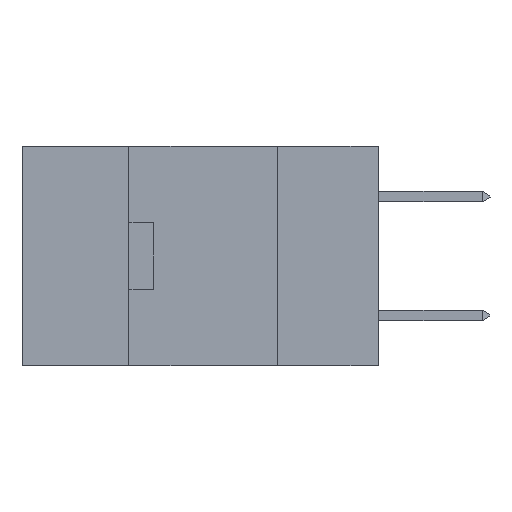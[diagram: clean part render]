
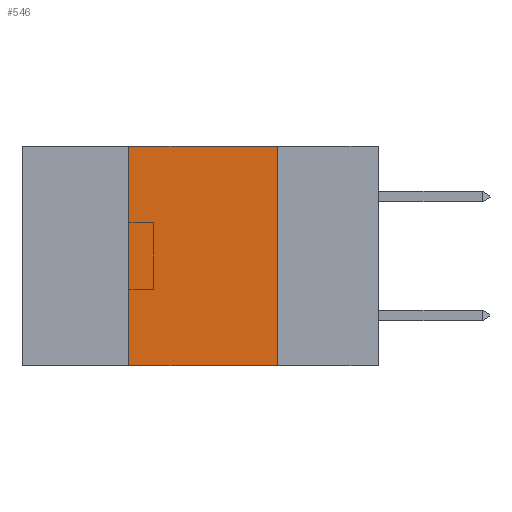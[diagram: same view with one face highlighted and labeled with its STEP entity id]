
A CAD part, left-side view. The second image highlights one B-rep face of the part: STEP entity #546.
In plain terms, the highlighted planar face has unit normal (-1, 0, 0).
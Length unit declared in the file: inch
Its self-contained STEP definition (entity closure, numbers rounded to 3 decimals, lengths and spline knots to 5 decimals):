
#224 = EDGE_CURVE ( 'NONE', #2833, #1646, #24307, .T. ) ;
#247 = VECTOR ( 'NONE', #17363, 39.37008 ) ;
#546 = ADVANCED_FACE ( 'NONE', ( #5704 ), #17321, .F. ) ;
#1470 = VERTEX_POINT ( 'NONE', #16471 ) ;
#1646 = VERTEX_POINT ( 'NONE', #10199 ) ;
#2113 = CARTESIAN_POINT ( 'NONE',  ( 0., 0.6, 0. ) ) ;
#2207 = DIRECTION ( 'NONE',  ( 0., -1., 0. ) ) ;
#2833 = VERTEX_POINT ( 'NONE', #9070 ) ;
#4577 = LINE ( 'NONE', #2113, #27231 ) ;
#5086 = AXIS2_PLACEMENT_3D ( 'NONE', #17224, #17189, #17125 ) ;
#5297 = ORIENTED_EDGE ( 'NONE', *, *, #15678, .F. ) ;
#5704 = FACE_OUTER_BOUND ( 'NONE', #21812, .T. ) ;
#6000 = ORIENTED_EDGE ( 'NONE', *, *, #16974, .F. ) ;
#7473 = DIRECTION ( 'NONE',  ( 0., 0., 1. ) ) ;
#9070 = CARTESIAN_POINT ( 'NONE',  ( 0., 0.42, -0.37 ) ) ;
#9795 = ORIENTED_EDGE ( 'NONE', *, *, #25012, .T. ) ;
#10057 = CARTESIAN_POINT ( 'NONE',  ( 0., 0.42, -0.37 ) ) ;
#10199 = CARTESIAN_POINT ( 'NONE',  ( 0., 0.42, 0. ) ) ;
#12077 = LINE ( 'NONE', #23946, #247 ) ;
#12909 = CARTESIAN_POINT ( 'NONE',  ( 0., 0.17, 0. ) ) ;
#15678 = EDGE_CURVE ( 'NONE', #1646, #18724, #4577, .T. ) ;
#16471 = CARTESIAN_POINT ( 'NONE',  ( 0., 0.17, -0.37 ) ) ;
#16974 = EDGE_CURVE ( 'NONE', #18724, #1470, #12077, .T. ) ;
#17125 = DIRECTION ( 'NONE',  ( 0., 0., -1. ) ) ;
#17189 = DIRECTION ( 'NONE',  ( 1., 0., 0. ) ) ;
#17224 = CARTESIAN_POINT ( 'NONE',  ( 0., 0.6, 0. ) ) ;
#17321 = PLANE ( 'NONE',  #5086 ) ;
#17363 = DIRECTION ( 'NONE',  ( 0., 0., -1. ) ) ;
#18535 = VECTOR ( 'NONE', #7473, 39.37008 ) ;
#18724 = VERTEX_POINT ( 'NONE', #12909 ) ;
#19442 = VECTOR ( 'NONE', #25407, 39.37008 ) ;
#20112 = LINE ( 'NONE', #23228, #19442 ) ;
#21812 = EDGE_LOOP ( 'NONE', ( #6000, #5297, #22202, #9795 ) ) ;
#22202 = ORIENTED_EDGE ( 'NONE', *, *, #224, .F. ) ;
#23228 = CARTESIAN_POINT ( 'NONE',  ( 0., 0.6, -0.37 ) ) ;
#23946 = CARTESIAN_POINT ( 'NONE',  ( 0., 0.17, -0.37 ) ) ;
#24307 = LINE ( 'NONE', #10057, #18535 ) ;
#25012 = EDGE_CURVE ( 'NONE', #2833, #1470, #20112, .T. ) ;
#25407 = DIRECTION ( 'NONE',  ( 0., -1., 0. ) ) ;
#27231 = VECTOR ( 'NONE', #2207, 39.37008 ) ;
